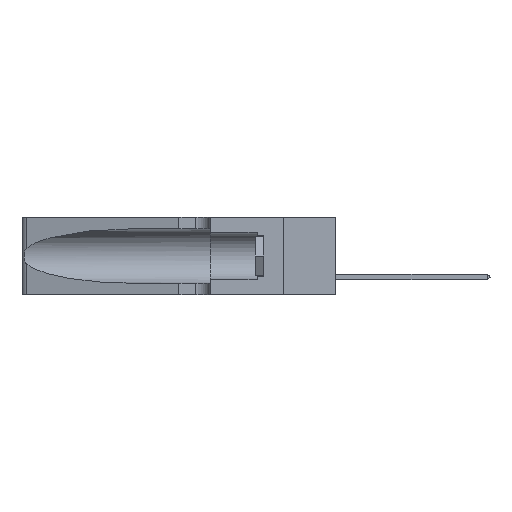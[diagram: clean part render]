
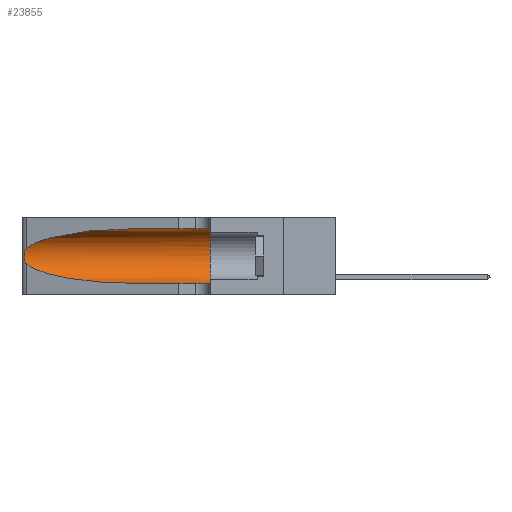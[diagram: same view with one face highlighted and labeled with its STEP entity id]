
A CAD part, left-side view. The second image highlights one B-rep face of the part: STEP entity #23855.
In plain terms, the highlighted cylindrical face has radius 3.308 mm (diameter 6.617 mm), a partial arc.
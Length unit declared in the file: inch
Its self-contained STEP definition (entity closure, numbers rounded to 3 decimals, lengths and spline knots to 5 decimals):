
#605 = CARTESIAN_POINT ( 'NONE',  ( 0.25639, 1.23184, 0.21858 ) ) ;
#1678 = ORIENTED_EDGE ( 'NONE', *, *, #10776, .T. ) ;
#2634 = B_SPLINE_CURVE_WITH_KNOTS ( 'NONE', 3,
 ( #7359, #22639, #605, #26916, #4997, #20266, #27014, #2983, #3082, #18376, #7459, #24908, #11815, #7171 ),
 .UNSPECIFIED., .F., .F.,
 ( 4, 2, 2, 2, 2, 2, 4 ),
 ( 0., 0.00027, 0.00053, 0.00107, 0.0016, 0.00187, 0.00214 ),
 .UNSPECIFIED. ) ;
#2983 = CARTESIAN_POINT ( 'NONE',  ( 0.26075, 1.23896, 0.178 ) ) ;
#3082 = CARTESIAN_POINT ( 'NONE',  ( 0.26017, 1.23833, 0.17102 ) ) ;
#3174 = AXIS2_PLACEMENT_3D ( 'NONE', #9346, #9644, #11736 ) ;
#3238 = CARTESIAN_POINT ( 'NONE',  ( 0.18966, 0.96281, 0.05475 ) ) ;
#3241 = DIRECTION ( 'NONE',  ( 0., -1., 0. ) ) ;
#4466 = CARTESIAN_POINT ( 'NONE',  ( 0.1305, 0.35, 0.05475 ) ) ;
#4480 = VERTEX_POINT ( 'NONE', #4466 ) ;
#4997 = CARTESIAN_POINT ( 'NONE',  ( 0.25854, 1.2359, 0.20912 ) ) ;
#5413 = DIRECTION ( 'NONE',  ( 0., -1., 0. ) ) ;
#5438 = CARTESIAN_POINT ( 'NONE',  ( 0.1305, 0.72297, 0.31525 ) ) ;
#5503 = DIRECTION ( 'NONE',  ( 0., 0., -1. ) ) ;
#6050 = ORIENTED_EDGE ( 'NONE', *, *, #18510, .T. ) ;
#6927 = VERTEX_POINT ( 'NONE', #7367 ) ;
#7153 = EDGE_CURVE ( 'NONE', #6927, #4480, #25702, .T. ) ;
#7171 = CARTESIAN_POINT ( 'NONE',  ( 0.25487, 1.22718, 0.14631 ) ) ;
#7177 = VERTEX_POINT ( 'NONE', #5438 ) ;
#7187 = CARTESIAN_POINT ( 'NONE',  ( 0.25487, 1.22718, 0.22369 ) ) ;
#7324 = ORIENTED_EDGE ( 'NONE', *, *, #11633, .T. ) ;
#7359 = CARTESIAN_POINT ( 'NONE',  ( 0.25487, 1.22718, 0.22369 ) ) ;
#7367 = CARTESIAN_POINT ( 'NONE',  ( 0.1305, 0.72297, 0.05475 ) ) ;
#7459 = CARTESIAN_POINT ( 'NONE',  ( 0.25789, 1.23486, 0.15765 ) ) ;
#7609 = CARTESIAN_POINT ( 'NONE',  ( 0.2373, 1.15595, 0.08982 ) ) ;
#8534 = CARTESIAN_POINT ( 'NONE',  ( 0.18966, 0.96281, 0.31525 ) ) ;
#9070 =( BOUNDED_CURVE ( )  B_SPLINE_CURVE ( 3, ( #23242, #7609, #3238, #14306 ),
 .UNSPECIFIED., .F., .F. ) 
 B_SPLINE_CURVE_WITH_KNOTS ( ( 4, 4 ),
 ( 3.44316, 4.71239 ),
 .UNSPECIFIED. ) 
 CURVE ( )  GEOMETRIC_REPRESENTATION_ITEM ( )  RATIONAL_B_SPLINE_CURVE ( ( 1., 0.87, 0.87, 1. ) ) 
 REPRESENTATION_ITEM ( '' )  );
#9175 = CARTESIAN_POINT ( 'NONE',  ( 0.2373, 1.15595, 0.28018 ) ) ;
#9346 = CARTESIAN_POINT ( 'NONE',  ( 0.1305, 0.35, 0.185 ) ) ;
#9644 = DIRECTION ( 'NONE',  ( 0., 1., 0. ) ) ;
#9665 = CARTESIAN_POINT ( 'NONE',  ( 0.25487, 1.22718, 0.14631 ) ) ;
#10776 = EDGE_CURVE ( 'NONE', #7177, #11428, #17538, .T. ) ;
#10943 = VERTEX_POINT ( 'NONE', #9665 ) ;
#11428 = VERTEX_POINT ( 'NONE', #25340 ) ;
#11562 = ORIENTED_EDGE ( 'NONE', *, *, #7153, .T. ) ;
#11633 = EDGE_CURVE ( 'NONE', #10943, #6927, #9070, .T. ) ;
#11736 = DIRECTION ( 'NONE',  ( 0., 0., 1. ) ) ;
#11815 = CARTESIAN_POINT ( 'NONE',  ( 0.25555, 1.22993, 0.14849 ) ) ;
#11870 = FACE_OUTER_BOUND ( 'NONE', #22034, .T. ) ;
#12794 = VERTEX_POINT ( 'NONE', #27409 ) ;
#12852 = LINE ( 'NONE', #20286, #17331 ) ;
#14306 = CARTESIAN_POINT ( 'NONE',  ( 0.1305, 0.72297, 0.05475 ) ) ;
#15339 = CYLINDRICAL_SURFACE ( 'NONE', #21032, 0.13025 ) ;
#15998 = DIRECTION ( 'NONE',  ( 0., -1., 0. ) ) ;
#16856 = EDGE_CURVE ( 'NONE', #12794, #4480, #21681, .T. ) ;
#17056 = ORIENTED_EDGE ( 'NONE', *, *, #25853, .F. ) ;
#17331 = VECTOR ( 'NONE', #15998, 39.37008 ) ;
#17538 =( BOUNDED_CURVE ( )  B_SPLINE_CURVE ( 3, ( #23623, #8534, #9175, #7187 ),
 .UNSPECIFIED., .F., .F. ) 
 B_SPLINE_CURVE_WITH_KNOTS ( ( 4, 4 ),
 ( 1.5708, 2.84003 ),
 .UNSPECIFIED. ) 
 CURVE ( )  GEOMETRIC_REPRESENTATION_ITEM ( )  RATIONAL_B_SPLINE_CURVE ( ( 1., 0.87, 0.87, 1. ) ) 
 REPRESENTATION_ITEM ( '' )  );
#18376 = CARTESIAN_POINT ( 'NONE',  ( 0.25856, 1.23593, 0.16098 ) ) ;
#18504 = CARTESIAN_POINT ( 'NONE',  ( 0.1305, 1.61858, 0.185 ) ) ;
#18510 = EDGE_CURVE ( 'NONE', #11428, #10943, #2634, .T. ) ;
#20266 = CARTESIAN_POINT ( 'NONE',  ( 0.26018, 1.23835, 0.19895 ) ) ;
#20286 = CARTESIAN_POINT ( 'NONE',  ( 0.1305, 1.61858, 0.31525 ) ) ;
#21032 = AXIS2_PLACEMENT_3D ( 'NONE', #18504, #5413, #5503 ) ;
#21681 = CIRCLE ( 'NONE', #3174, 0.13025 ) ;
#21955 = VECTOR ( 'NONE', #3241, 39.37008 ) ;
#22034 = EDGE_LOOP ( 'NONE', ( #1678, #6050, #7324, #11562, #24281, #17056 ) ) ;
#22639 = CARTESIAN_POINT ( 'NONE',  ( 0.25555, 1.22994, 0.2215 ) ) ;
#23242 = CARTESIAN_POINT ( 'NONE',  ( 0.25487, 1.22718, 0.14631 ) ) ;
#23623 = CARTESIAN_POINT ( 'NONE',  ( 0.1305, 0.72297, 0.31525 ) ) ;
#23855 = ADVANCED_FACE ( 'NONE', ( #11870 ), #15339, .F. ) ;
#24281 = ORIENTED_EDGE ( 'NONE', *, *, #16856, .F. ) ;
#24908 = CARTESIAN_POINT ( 'NONE',  ( 0.25639, 1.23186, 0.15144 ) ) ;
#25340 = CARTESIAN_POINT ( 'NONE',  ( 0.25487, 1.22718, 0.22369 ) ) ;
#25702 = LINE ( 'NONE', #26872, #21955 ) ;
#25853 = EDGE_CURVE ( 'NONE', #7177, #12794, #12852, .T. ) ;
#26872 = CARTESIAN_POINT ( 'NONE',  ( 0.1305, 1.61858, 0.05475 ) ) ;
#26916 = CARTESIAN_POINT ( 'NONE',  ( 0.25787, 1.23484, 0.2124 ) ) ;
#27014 = CARTESIAN_POINT ( 'NONE',  ( 0.26075, 1.23896, 0.19203 ) ) ;
#27409 = CARTESIAN_POINT ( 'NONE',  ( 0.1305, 0.35, 0.31525 ) ) ;
